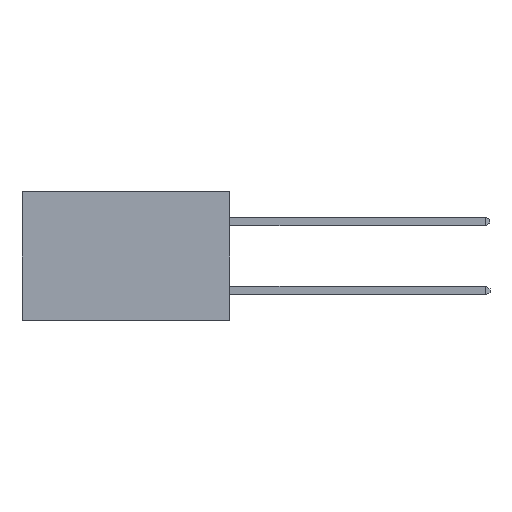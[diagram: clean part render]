
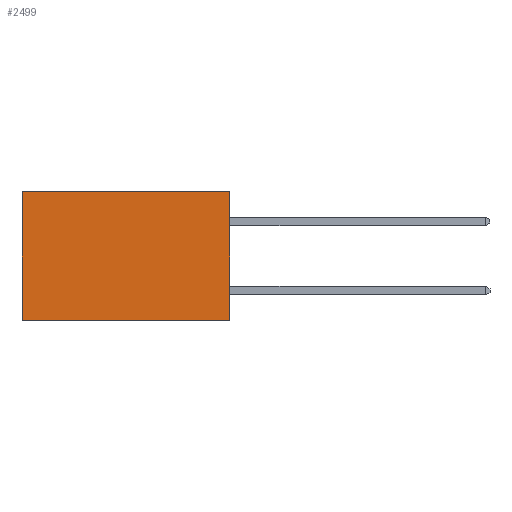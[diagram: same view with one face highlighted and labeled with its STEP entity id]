
A CAD part, left-side view. The second image highlights one B-rep face of the part: STEP entity #2499.
In plain terms, the highlighted planar face has unit normal (-1, 0, 0).
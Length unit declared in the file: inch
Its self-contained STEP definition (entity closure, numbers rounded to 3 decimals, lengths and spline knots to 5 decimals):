
#104 = ORIENTED_EDGE ( 'NONE', *, *, #8385, .F. ) ;
#428 = CARTESIAN_POINT ( 'NONE',  ( 0.2615, 0.6, 0. ) ) ;
#435 = VERTEX_POINT ( 'NONE', #7304 ) ;
#487 = VECTOR ( 'NONE', #4260, 39.37008 ) ;
#644 = ORIENTED_EDGE ( 'NONE', *, *, #5389, .F. ) ;
#732 = VERTEX_POINT ( 'NONE', #5136 ) ;
#800 = EDGE_LOOP ( 'NONE', ( #5926, #104, #644, #8343 ) ) ;
#1180 = VECTOR ( 'NONE', #4424, 39.37008 ) ;
#1284 = VECTOR ( 'NONE', #8948, 39.37008 ) ;
#1796 = DIRECTION ( 'NONE',  ( 0., 1., 0. ) ) ;
#1861 = CARTESIAN_POINT ( 'NONE',  ( 0.2615, 0., 0. ) ) ;
#2047 = LINE ( 'NONE', #1861, #8979 ) ;
#2146 = AXIS2_PLACEMENT_3D ( 'NONE', #7756, #7504, #7468 ) ;
#2499 = ADVANCED_FACE ( 'NONE', ( #6224 ), #7609, .F. ) ;
#3474 = CARTESIAN_POINT ( 'NONE',  ( 0.2615, 0., -0.37 ) ) ;
#3746 = EDGE_CURVE ( 'NONE', #4292, #435, #6949, .T. ) ;
#3782 = CARTESIAN_POINT ( 'NONE',  ( 0.2615, 0., 0. ) ) ;
#3843 = VERTEX_POINT ( 'NONE', #3782 ) ;
#4114 = EDGE_CURVE ( 'NONE', #3843, #4292, #2047, .T. ) ;
#4260 = DIRECTION ( 'NONE',  ( 0., 0., -1. ) ) ;
#4292 = VERTEX_POINT ( 'NONE', #428 ) ;
#4333 = CARTESIAN_POINT ( 'NONE',  ( 0.2615, 0., -0.37 ) ) ;
#4422 = CARTESIAN_POINT ( 'NONE',  ( 0.2615, 0.6, -0.37 ) ) ;
#4424 = DIRECTION ( 'NONE',  ( 0., 0., -1. ) ) ;
#5136 = CARTESIAN_POINT ( 'NONE',  ( 0.2615, 0., -0.37 ) ) ;
#5389 = EDGE_CURVE ( 'NONE', #3843, #732, #7907, .T. ) ;
#5926 = ORIENTED_EDGE ( 'NONE', *, *, #3746, .T. ) ;
#6224 = FACE_OUTER_BOUND ( 'NONE', #800, .T. ) ;
#6949 = LINE ( 'NONE', #4422, #1180 ) ;
#7028 = LINE ( 'NONE', #3474, #1284 ) ;
#7304 = CARTESIAN_POINT ( 'NONE',  ( 0.2615, 0.6, -0.37 ) ) ;
#7468 = DIRECTION ( 'NONE',  ( 0., 0., -1. ) ) ;
#7504 = DIRECTION ( 'NONE',  ( 1., 0., 0. ) ) ;
#7609 = PLANE ( 'NONE',  #2146 ) ;
#7756 = CARTESIAN_POINT ( 'NONE',  ( 0.2615, 0., -0.37 ) ) ;
#7907 = LINE ( 'NONE', #4333, #487 ) ;
#8343 = ORIENTED_EDGE ( 'NONE', *, *, #4114, .T. ) ;
#8385 = EDGE_CURVE ( 'NONE', #732, #435, #7028, .T. ) ;
#8948 = DIRECTION ( 'NONE',  ( 0., 1., 0. ) ) ;
#8979 = VECTOR ( 'NONE', #1796, 39.37008 ) ;
